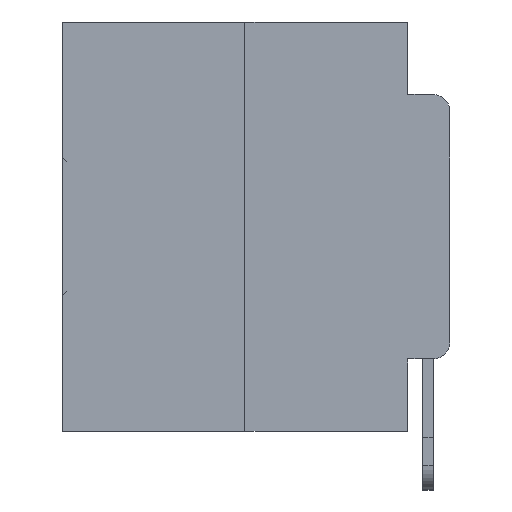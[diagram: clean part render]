
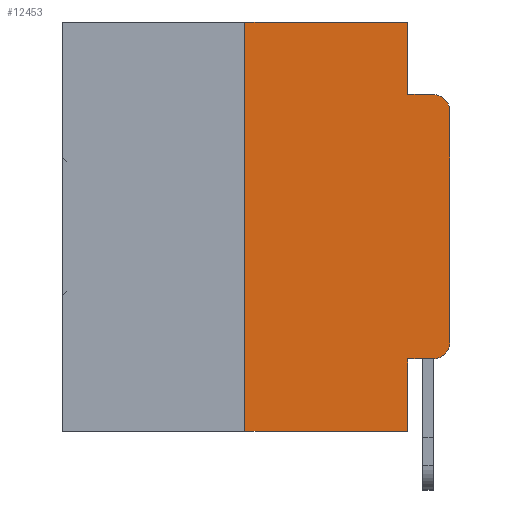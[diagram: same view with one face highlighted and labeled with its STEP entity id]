
A CAD part, left-side view. The second image highlights one B-rep face of the part: STEP entity #12453.
In plain terms, the highlighted planar face has unit normal (-1, 0, 0).
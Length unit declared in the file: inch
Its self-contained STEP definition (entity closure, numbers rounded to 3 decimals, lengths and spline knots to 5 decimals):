
#270 = ORIENTED_EDGE ( 'NONE', *, *, #15541, .T. ) ;
#336 = CARTESIAN_POINT ( 'NONE',  ( 0., 0.051, -0.4115 ) ) ;
#479 = LINE ( 'NONE', #6052, #20554 ) ;
#492 = CARTESIAN_POINT ( 'NONE',  ( 0., 0.25, 0. ) ) ;
#1077 = CARTESIAN_POINT ( 'NONE',  ( 0., 0.473, 0. ) ) ;
#1103 = CARTESIAN_POINT ( 'NONE',  ( 0., 0., -0.1085 ) ) ;
#1126 = DIRECTION ( 'NONE',  ( 0., 0., -1. ) ) ;
#1944 = CARTESIAN_POINT ( 'NONE',  ( 0., 0.051, -0.4115 ) ) ;
#2184 = LINE ( 'NONE', #7636, #27441 ) ;
#2413 = EDGE_CURVE ( 'NONE', #4539, #29028, #25416, .T. ) ;
#3145 = FACE_OUTER_BOUND ( 'NONE', #10459, .T. ) ;
#3200 = CARTESIAN_POINT ( 'NONE',  ( 0., 0.02, -0.0885 ) ) ;
#3201 = VECTOR ( 'NONE', #30291, 39.37008 ) ;
#3340 = LINE ( 'NONE', #20555, #28438 ) ;
#4239 = DIRECTION ( 'NONE',  ( 0., 0., -1. ) ) ;
#4539 = VERTEX_POINT ( 'NONE', #23708 ) ;
#4688 = VERTEX_POINT ( 'NONE', #12190 ) ;
#5639 = VERTEX_POINT ( 'NONE', #1103 ) ;
#6002 = VECTOR ( 'NONE', #22370, 39.37008 ) ;
#6052 = CARTESIAN_POINT ( 'NONE',  ( 0., 0.473, -0.5 ) ) ;
#6935 = CARTESIAN_POINT ( 'NONE',  ( 0., 0.051, -0.5 ) ) ;
#7636 = CARTESIAN_POINT ( 'NONE',  ( 0., 0., 0. ) ) ;
#8300 = DIRECTION ( 'NONE',  ( 0., 0., -1. ) ) ;
#8690 = ORIENTED_EDGE ( 'NONE', *, *, #24496, .F. ) ;
#8861 = EDGE_CURVE ( 'NONE', #5639, #29028, #28483, .T. ) ;
#9313 = EDGE_CURVE ( 'NONE', #16910, #28703, #20142, .T. ) ;
#9772 = CARTESIAN_POINT ( 'NONE',  ( 0., 0.051, 0. ) ) ;
#9801 = VECTOR ( 'NONE', #4239, 39.37008 ) ;
#9903 = EDGE_CURVE ( 'NONE', #4688, #31122, #22227, .T. ) ;
#10100 = DIRECTION ( 'NONE',  ( 0., 0., 1. ) ) ;
#10459 = EDGE_LOOP ( 'NONE', ( #270, #23965, #14607, #8690, #24294, #23282, #20011, #14616, #20665, #17447 ) ) ;
#12190 = CARTESIAN_POINT ( 'NONE',  ( 0., 0.25, -0.5 ) ) ;
#12453 = ADVANCED_FACE ( 'NONE', ( #3145 ), #28010, .F. ) ;
#12835 = VECTOR ( 'NONE', #22805, 39.37008 ) ;
#13818 = CARTESIAN_POINT ( 'NONE',  ( 0., 0.473, 0. ) ) ;
#13897 = DIRECTION ( 'NONE',  ( -1., 0., 0. ) ) ;
#14143 = EDGE_CURVE ( 'NONE', #4688, #25898, #479, .T. ) ;
#14290 = EDGE_CURVE ( 'NONE', #28703, #16637, #31005, .T. ) ;
#14313 = DIRECTION ( 'NONE',  ( -1., 0., 0. ) ) ;
#14607 = ORIENTED_EDGE ( 'NONE', *, *, #2413, .F. ) ;
#14616 = ORIENTED_EDGE ( 'NONE', *, *, #16578, .F. ) ;
#15541 = EDGE_CURVE ( 'NONE', #16637, #5639, #2184, .T. ) ;
#15890 = VECTOR ( 'NONE', #18210, 39.37008 ) ;
#15992 = CARTESIAN_POINT ( 'NONE',  ( 0., 0., -0.3915 ) ) ;
#16292 = DIRECTION ( 'NONE',  ( 1., 0., 0. ) ) ;
#16578 = EDGE_CURVE ( 'NONE', #16910, #25898, #3340, .T. ) ;
#16581 = LINE ( 'NONE', #1077, #3201 ) ;
#16637 = VERTEX_POINT ( 'NONE', #15992 ) ;
#16910 = VERTEX_POINT ( 'NONE', #1944 ) ;
#17252 = CARTESIAN_POINT ( 'NONE',  ( 0., 0.02, -0.4115 ) ) ;
#17447 = ORIENTED_EDGE ( 'NONE', *, *, #14290, .T. ) ;
#17803 = AXIS2_PLACEMENT_3D ( 'NONE', #28069, #13897, #30415 ) ;
#18210 = DIRECTION ( 'NONE',  ( 0., 0., 1. ) ) ;
#19195 = CARTESIAN_POINT ( 'NONE',  ( 0., 0.051, 0. ) ) ;
#19379 = AXIS2_PLACEMENT_3D ( 'NONE', #28475, #14313, #30828 ) ;
#20011 = ORIENTED_EDGE ( 'NONE', *, *, #14143, .T. ) ;
#20142 = LINE ( 'NONE', #336, #12835 ) ;
#20554 = VECTOR ( 'NONE', #23156, 39.37008 ) ;
#20555 = CARTESIAN_POINT ( 'NONE',  ( 0., 0.051, 0. ) ) ;
#20665 = ORIENTED_EDGE ( 'NONE', *, *, #9313, .T. ) ;
#21862 = EDGE_CURVE ( 'NONE', #31122, #28610, #16581, .T. ) ;
#21920 = CARTESIAN_POINT ( 'NONE',  ( 0., 0.051, -0.0885 ) ) ;
#22227 = LINE ( 'NONE', #492, #15890 ) ;
#22370 = DIRECTION ( 'NONE',  ( 0., -1., 0. ) ) ;
#22494 = AXIS2_PLACEMENT_3D ( 'NONE', #13818, #16292, #1126 ) ;
#22805 = DIRECTION ( 'NONE',  ( 0., -1., 0. ) ) ;
#23156 = DIRECTION ( 'NONE',  ( 0., -1., 0. ) ) ;
#23282 = ORIENTED_EDGE ( 'NONE', *, *, #9903, .F. ) ;
#23495 = LINE ( 'NONE', #19195, #9801 ) ;
#23708 = CARTESIAN_POINT ( 'NONE',  ( 0., 0.051, -0.0885 ) ) ;
#23965 = ORIENTED_EDGE ( 'NONE', *, *, #8861, .T. ) ;
#24294 = ORIENTED_EDGE ( 'NONE', *, *, #21862, .F. ) ;
#24496 = EDGE_CURVE ( 'NONE', #28610, #4539, #23495, .T. ) ;
#25416 = LINE ( 'NONE', #21920, #6002 ) ;
#25898 = VERTEX_POINT ( 'NONE', #6935 ) ;
#27441 = VECTOR ( 'NONE', #10100, 39.37008 ) ;
#28010 = PLANE ( 'NONE',  #22494 ) ;
#28069 = CARTESIAN_POINT ( 'NONE',  ( 0., 0.02, -0.1085 ) ) ;
#28438 = VECTOR ( 'NONE', #8300, 39.37008 ) ;
#28475 = CARTESIAN_POINT ( 'NONE',  ( 0., 0.02, -0.3915 ) ) ;
#28483 = CIRCLE ( 'NONE', #17803, 0.02 ) ;
#28610 = VERTEX_POINT ( 'NONE', #9772 ) ;
#28703 = VERTEX_POINT ( 'NONE', #17252 ) ;
#28742 = CARTESIAN_POINT ( 'NONE',  ( 0., 0.25, 0. ) ) ;
#29028 = VERTEX_POINT ( 'NONE', #3200 ) ;
#30291 = DIRECTION ( 'NONE',  ( 0., -1., 0. ) ) ;
#30415 = DIRECTION ( 'NONE',  ( 0., 0., -1. ) ) ;
#30828 = DIRECTION ( 'NONE',  ( 0., 0., -1. ) ) ;
#31005 = CIRCLE ( 'NONE', #19379, 0.02 ) ;
#31122 = VERTEX_POINT ( 'NONE', #28742 ) ;
